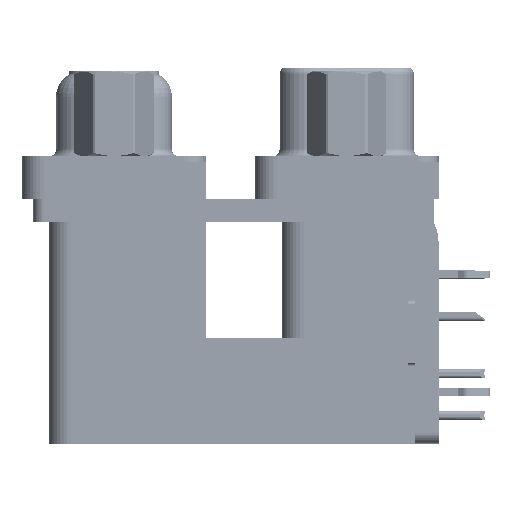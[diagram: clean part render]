
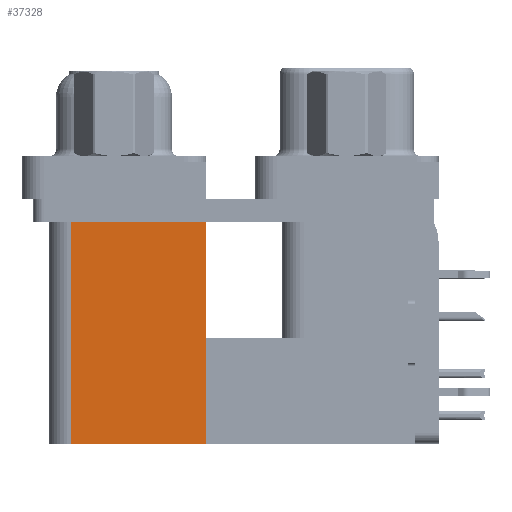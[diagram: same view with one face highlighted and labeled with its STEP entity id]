
A CAD part, left-side view. The second image highlights one B-rep face of the part: STEP entity #37328.
In plain terms, the highlighted planar face has unit normal (-1, 0, 0).
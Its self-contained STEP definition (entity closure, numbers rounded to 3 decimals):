
#142 = ORIENTED_EDGE ( 'NONE', *, *, #54595, .F. ) ;
#2793 = EDGE_CURVE ( 'NONE', #12425, #20365, #8063, .T. ) ;
#8063 = LINE ( 'NONE', #61397, #44554 ) ;
#8688 = DIRECTION ( 'NONE',  ( 0., 1., 0. ) ) ;
#10699 = CARTESIAN_POINT ( 'NONE',  ( 3.7, 9.6, -19.2 ) ) ;
#11167 = CARTESIAN_POINT ( 'NONE',  ( 3.7, 9.6, -19.2 ) ) ;
#12425 = VERTEX_POINT ( 'NONE', #10699 ) ;
#13279 = CARTESIAN_POINT ( 'NONE',  ( 3.7, 18.8, -19.2 ) ) ;
#14445 = EDGE_CURVE ( 'NONE', #61050, #32661, #14729, .T. ) ;
#14558 = AXIS2_PLACEMENT_3D ( 'NONE', #18337, #45799, #36298 ) ;
#14729 = LINE ( 'NONE', #34890, #39499 ) ;
#15612 = LINE ( 'NONE', #11167, #26951 ) ;
#17066 = FACE_OUTER_BOUND ( 'NONE', #49012, .T. ) ;
#18337 = CARTESIAN_POINT ( 'NONE',  ( 3.7, 9.6, -19.2 ) ) ;
#18582 = LINE ( 'NONE', #23917, #33930 ) ;
#20365 = VERTEX_POINT ( 'NONE', #13279 ) ;
#23917 = CARTESIAN_POINT ( 'NONE',  ( 3.7, 18.8, -19.2 ) ) ;
#25114 = EDGE_CURVE ( 'NONE', #12425, #61050, #15612, .T. ) ;
#25396 = ORIENTED_EDGE ( 'NONE', *, *, #25114, .T. ) ;
#26951 = VECTOR ( 'NONE', #49719, 1000. ) ;
#32046 = CARTESIAN_POINT ( 'NONE',  ( 3.7, 18.8, -2.5 ) ) ;
#32661 = VERTEX_POINT ( 'NONE', #32046 ) ;
#33930 = VECTOR ( 'NONE', #43198, 1000. ) ;
#33977 = DIRECTION ( 'NONE',  ( 0., 1., 0. ) ) ;
#34890 = CARTESIAN_POINT ( 'NONE',  ( 3.7, 9.6, -2.5 ) ) ;
#36298 = DIRECTION ( 'NONE',  ( 0., 0., -1. ) ) ;
#37328 = ADVANCED_FACE ( 'NONE', ( #17066 ), #41694, .F. ) ;
#39499 = VECTOR ( 'NONE', #33977, 1000. ) ;
#41694 = PLANE ( 'NONE',  #14558 ) ;
#43198 = DIRECTION ( 'NONE',  ( 0., 0., 1. ) ) ;
#44554 = VECTOR ( 'NONE', #8688, 1000. ) ;
#45799 = DIRECTION ( 'NONE',  ( 1., 0., 0. ) ) ;
#46833 = CARTESIAN_POINT ( 'NONE',  ( 3.7, 9.6, -2.5 ) ) ;
#49012 = EDGE_LOOP ( 'NONE', ( #60435, #142, #54430, #25396 ) ) ;
#49719 = DIRECTION ( 'NONE',  ( 0., 0., 1. ) ) ;
#54430 = ORIENTED_EDGE ( 'NONE', *, *, #2793, .F. ) ;
#54595 = EDGE_CURVE ( 'NONE', #20365, #32661, #18582, .T. ) ;
#60435 = ORIENTED_EDGE ( 'NONE', *, *, #14445, .T. ) ;
#61050 = VERTEX_POINT ( 'NONE', #46833 ) ;
#61397 = CARTESIAN_POINT ( 'NONE',  ( 3.7, 9.6, -19.2 ) ) ;
